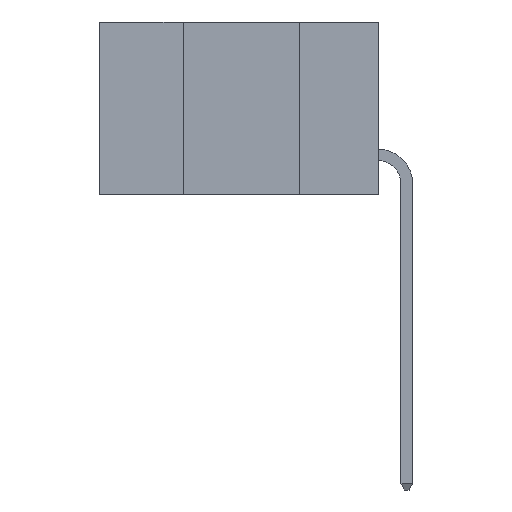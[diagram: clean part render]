
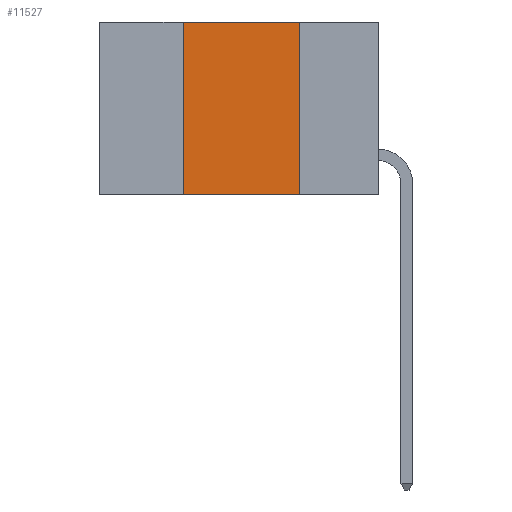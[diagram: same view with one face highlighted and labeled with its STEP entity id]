
A CAD part, left-side view. The second image highlights one B-rep face of the part: STEP entity #11527.
In plain terms, the highlighted planar face has unit normal (-1, 0, 0).
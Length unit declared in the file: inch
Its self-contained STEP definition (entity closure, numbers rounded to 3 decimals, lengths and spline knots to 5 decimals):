
#39 = ORIENTED_EDGE ( 'NONE', *, *, #11494, .T. ) ;
#361 = VERTEX_POINT ( 'NONE', #10625 ) ;
#891 = DIRECTION ( 'NONE',  ( 0., -1., 0. ) ) ;
#1431 = VERTEX_POINT ( 'NONE', #9026 ) ;
#1476 = ORIENTED_EDGE ( 'NONE', *, *, #12344, .F. ) ;
#1503 = ORIENTED_EDGE ( 'NONE', *, *, #13186, .F. ) ;
#1517 = DIRECTION ( 'NONE',  ( 0., -1., 0. ) ) ;
#1633 = ORIENTED_EDGE ( 'NONE', *, *, #14009, .F. ) ;
#1953 = AXIS2_PLACEMENT_3D ( 'NONE', #14478, #15706, #8230 ) ;
#2413 = VERTEX_POINT ( 'NONE', #8569 ) ;
#2630 = CARTESIAN_POINT ( 'NONE',  ( 0., 0.17, 0. ) ) ;
#3886 = VECTOR ( 'NONE', #891, 39.37008 ) ;
#4540 = LINE ( 'NONE', #10663, #10963 ) ;
#4575 = CARTESIAN_POINT ( 'NONE',  ( 0., 0.42, -0.37 ) ) ;
#5441 = DIRECTION ( 'NONE',  ( 0., 0., -1. ) ) ;
#5627 = PLANE ( 'NONE',  #1953 ) ;
#5877 = VERTEX_POINT ( 'NONE', #2630 ) ;
#5878 = DIRECTION ( 'NONE',  ( 0., 0., 1. ) ) ;
#5921 = EDGE_LOOP ( 'NONE', ( #1633, #1503, #1476, #39 ) ) ;
#7383 = LINE ( 'NONE', #13846, #3886 ) ;
#7587 = VECTOR ( 'NONE', #5878, 39.37008 ) ;
#7999 = LINE ( 'NONE', #4575, #7587 ) ;
#8230 = DIRECTION ( 'NONE',  ( 0., 0., -1. ) ) ;
#8569 = CARTESIAN_POINT ( 'NONE',  ( 0., 0.42, 0. ) ) ;
#9026 = CARTESIAN_POINT ( 'NONE',  ( 0., 0.17, -0.37 ) ) ;
#9516 = VECTOR ( 'NONE', #5441, 39.37008 ) ;
#10625 = CARTESIAN_POINT ( 'NONE',  ( 0., 0.42, -0.37 ) ) ;
#10663 = CARTESIAN_POINT ( 'NONE',  ( 0., 0.6, -0.37 ) ) ;
#10963 = VECTOR ( 'NONE', #1517, 39.37008 ) ;
#11494 = EDGE_CURVE ( 'NONE', #361, #1431, #4540, .T. ) ;
#11527 = ADVANCED_FACE ( 'NONE', ( #13905 ), #5627, .F. ) ;
#12344 = EDGE_CURVE ( 'NONE', #361, #2413, #7999, .T. ) ;
#12872 = LINE ( 'NONE', #14293, #9516 ) ;
#13186 = EDGE_CURVE ( 'NONE', #2413, #5877, #7383, .T. ) ;
#13846 = CARTESIAN_POINT ( 'NONE',  ( 0., 0.6, 0. ) ) ;
#13905 = FACE_OUTER_BOUND ( 'NONE', #5921, .T. ) ;
#14009 = EDGE_CURVE ( 'NONE', #5877, #1431, #12872, .T. ) ;
#14293 = CARTESIAN_POINT ( 'NONE',  ( 0., 0.17, -0.37 ) ) ;
#14478 = CARTESIAN_POINT ( 'NONE',  ( 0., 0.6, 0. ) ) ;
#15706 = DIRECTION ( 'NONE',  ( 1., 0., 0. ) ) ;
